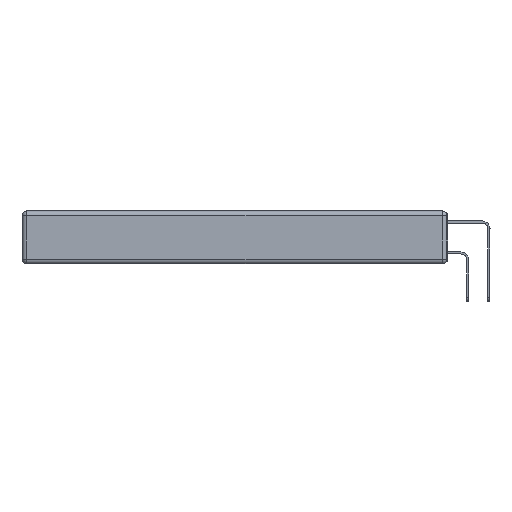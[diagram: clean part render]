
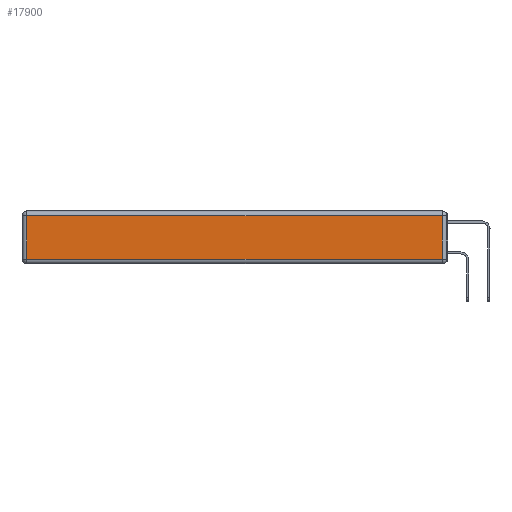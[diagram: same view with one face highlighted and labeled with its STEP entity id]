
A CAD part, left-side view. The second image highlights one B-rep face of the part: STEP entity #17900.
In plain terms, the highlighted planar face has unit normal (-1, 0, 0).
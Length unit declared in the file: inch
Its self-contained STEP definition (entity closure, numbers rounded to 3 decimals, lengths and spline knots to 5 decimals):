
#444 = FACE_OUTER_BOUND ( 'NONE', #14438, .T. ) ;
#1097 = EDGE_CURVE ( 'NONE', #8124, #20113, #19091, .T. ) ;
#3652 = DIRECTION ( 'NONE',  ( -1., 0., 0. ) ) ;
#3930 = ORIENTED_EDGE ( 'NONE', *, *, #13598, .T. ) ;
#6077 = LINE ( 'NONE', #26399, #8181 ) ;
#8094 = LINE ( 'NONE', #14955, #11622 ) ;
#8124 = VERTEX_POINT ( 'NONE', #8791 ) ;
#8181 = VECTOR ( 'NONE', #21965, 39.37008 ) ;
#8409 = CARTESIAN_POINT ( 'NONE',  ( 0., 0., -0.343 ) ) ;
#8579 = EDGE_CURVE ( 'NONE', #21885, #16416, #8094, .T. ) ;
#8791 = CARTESIAN_POINT ( 'NONE',  ( 0., 2.72, -0.313 ) ) ;
#9869 = AXIS2_PLACEMENT_3D ( 'NONE', #8409, #3652, #24418 ) ;
#11461 = ORIENTED_EDGE ( 'NONE', *, *, #21703, .T. ) ;
#11622 = VECTOR ( 'NONE', #23989, 39.37008 ) ;
#12245 = ORIENTED_EDGE ( 'NONE', *, *, #8579, .T. ) ;
#13470 = VECTOR ( 'NONE', #21953, 39.37008 ) ;
#13598 = EDGE_CURVE ( 'NONE', #16416, #8124, #14522, .T. ) ;
#14438 = EDGE_LOOP ( 'NONE', ( #15182, #11461, #12245, #3930 ) ) ;
#14522 = LINE ( 'NONE', #21130, #27270 ) ;
#14955 = CARTESIAN_POINT ( 'NONE',  ( 0., 2.75, -0.03 ) ) ;
#15182 = ORIENTED_EDGE ( 'NONE', *, *, #1097, .T. ) ;
#15192 = PLANE ( 'NONE',  #9869 ) ;
#16416 = VERTEX_POINT ( 'NONE', #18888 ) ;
#17900 = ADVANCED_FACE ( 'NONE', ( #444 ), #15192, .T. ) ;
#18888 = CARTESIAN_POINT ( 'NONE',  ( 0., 2.72, -0.03 ) ) ;
#19091 = LINE ( 'NONE', #19568, #13470 ) ;
#19568 = CARTESIAN_POINT ( 'NONE',  ( 0., 0., -0.313 ) ) ;
#20113 = VERTEX_POINT ( 'NONE', #20810 ) ;
#20810 = CARTESIAN_POINT ( 'NONE',  ( 0., 0.03, -0.313 ) ) ;
#21130 = CARTESIAN_POINT ( 'NONE',  ( 0., 2.72, -0.343 ) ) ;
#21703 = EDGE_CURVE ( 'NONE', #20113, #21885, #6077, .T. ) ;
#21885 = VERTEX_POINT ( 'NONE', #26800 ) ;
#21953 = DIRECTION ( 'NONE',  ( 0., -1., 0. ) ) ;
#21965 = DIRECTION ( 'NONE',  ( 0., 0., 1. ) ) ;
#23989 = DIRECTION ( 'NONE',  ( 0., 1., 0. ) ) ;
#24418 = DIRECTION ( 'NONE',  ( 0., 0., 1. ) ) ;
#26399 = CARTESIAN_POINT ( 'NONE',  ( 0., 0.03, -0.343 ) ) ;
#26800 = CARTESIAN_POINT ( 'NONE',  ( 0., 0.03, -0.03 ) ) ;
#27270 = VECTOR ( 'NONE', #28022, 39.37008 ) ;
#28022 = DIRECTION ( 'NONE',  ( 0., 0., -1. ) ) ;
